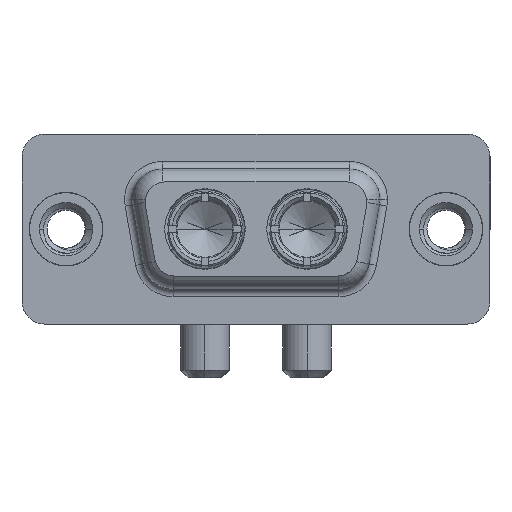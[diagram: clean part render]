
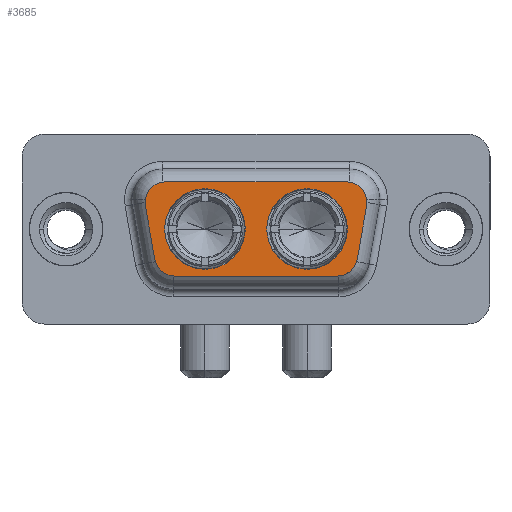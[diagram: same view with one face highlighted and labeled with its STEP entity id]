
A CAD part, top view. The second image highlights one B-rep face of the part: STEP entity #3685.
In plain terms, the highlighted planar face has unit normal (0, 0, 1).
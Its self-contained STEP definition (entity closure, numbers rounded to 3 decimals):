
#141 = CIRCLE ( 'NONE', #6974, 2.65 ) ;
#162 = VERTEX_POINT ( 'NONE', #2489 ) ;
#272 = EDGE_CURVE ( 'NONE', #11882, #10752, #141, .T. ) ;
#481 = AXIS2_PLACEMENT_3D ( 'NONE', #8998, #1704, #1577 ) ;
#513 = VERTEX_POINT ( 'NONE', #658 ) ;
#582 = EDGE_CURVE ( 'NONE', #7479, #8769, #7341, .T. ) ;
#658 = CARTESIAN_POINT ( 'NONE',  ( 17.833, -3.1, 6.2 ) ) ;
#794 = ORIENTED_EDGE ( 'NONE', *, *, #5328, .T. ) ;
#813 = EDGE_CURVE ( 'NONE', #10752, #11882, #9710, .T. ) ;
#940 = VERTEX_POINT ( 'NONE', #2238 ) ;
#1012 = CARTESIAN_POINT ( 'NONE',  ( 19.779, 1.516, 6.2 ) ) ;
#1133 = CARTESIAN_POINT ( 'NONE',  ( 6.55, 3.1, 6.2 ) ) ;
#1221 = EDGE_CURVE ( 'NONE', #513, #4350, #10902, .T. ) ;
#1240 = DIRECTION ( 'NONE',  ( 0., 0., 1. ) ) ;
#1475 = ORIENTED_EDGE ( 'NONE', *, *, #582, .T. ) ;
#1577 = DIRECTION ( 'NONE',  ( 1., 0., 0. ) ) ;
#1593 = LINE ( 'NONE', #2452, #9607 ) ;
#1704 = DIRECTION ( 'NONE',  ( 0., 0., 1. ) ) ;
#1776 = DIRECTION ( 'NONE',  ( -1., 0., 0. ) ) ;
#1839 = CARTESIAN_POINT ( 'NONE',  ( 19.162, -1.984, 6.2 ) ) ;
#2238 = CARTESIAN_POINT ( 'NONE',  ( 5.838, -1.984, 6.2 ) ) ;
#2259 = ORIENTED_EDGE ( 'NONE', *, *, #1221, .T. ) ;
#2313 = CARTESIAN_POINT ( 'NONE',  ( 18.51, 0., 6.2 ) ) ;
#2421 = AXIS2_PLACEMENT_3D ( 'NONE', #9107, #5480, #8126 ) ;
#2452 = CARTESIAN_POINT ( 'NONE',  ( 17.833, -3.1, 6.2 ) ) ;
#2489 = CARTESIAN_POINT ( 'NONE',  ( 5.221, 1.516, 6.2 ) ) ;
#2652 = CARTESIAN_POINT ( 'NONE',  ( 5.2, 1.75, 6.2 ) ) ;
#2676 = PLANE ( 'NONE',  #7298 ) ;
#2788 = CARTESIAN_POINT ( 'NONE',  ( 11.79, 0., 6.2 ) ) ;
#2874 = DIRECTION ( 'NONE',  ( 0., 0., 1. ) ) ;
#2906 = EDGE_CURVE ( 'NONE', #5602, #3617, #6152, .T. ) ;
#3051 = DIRECTION ( 'NONE',  ( 1., 0., 0. ) ) ;
#3231 = ORIENTED_EDGE ( 'NONE', *, *, #4166, .T. ) ;
#3270 = EDGE_LOOP ( 'NONE', ( #8296, #8407 ) ) ;
#3288 = CARTESIAN_POINT ( 'NONE',  ( 7.167, -3.1, 6.2 ) ) ;
#3304 = DIRECTION ( 'NONE',  ( 1., 0., 0. ) ) ;
#3306 = ORIENTED_EDGE ( 'NONE', *, *, #4454, .T. ) ;
#3411 = CARTESIAN_POINT ( 'NONE',  ( 7.167, -1.75, 6.2 ) ) ;
#3592 = AXIS2_PLACEMENT_3D ( 'NONE', #3713, #5357, #3051 ) ;
#3617 = VERTEX_POINT ( 'NONE', #2313 ) ;
#3652 = FACE_BOUND ( 'NONE', #3270, .T. ) ;
#3664 = EDGE_LOOP ( 'NONE', ( #5469, #6252 ) ) ;
#3685 = ADVANCED_FACE ( 'NONE', ( #3652, #12069, #4448 ), #2676, .F. ) ;
#3713 = CARTESIAN_POINT ( 'NONE',  ( 6.55, 1.75, 6.2 ) ) ;
#3870 = CARTESIAN_POINT ( 'NONE',  ( 17.833, -1.75, 6.2 ) ) ;
#3876 = CARTESIAN_POINT ( 'NONE',  ( 6.49, 0., 6.2 ) ) ;
#3910 = CIRCLE ( 'NONE', #6471, 1.35 ) ;
#4017 = CARTESIAN_POINT ( 'NONE',  ( 7.167, -1.75, 6.2 ) ) ;
#4047 = EDGE_CURVE ( 'NONE', #12054, #162, #3910, .T. ) ;
#4166 = EDGE_CURVE ( 'NONE', #10461, #513, #1593, .T. ) ;
#4350 = VERTEX_POINT ( 'NONE', #1839 ) ;
#4440 = VECTOR ( 'NONE', #9411, 1000. ) ;
#4448 = FACE_OUTER_BOUND ( 'NONE', #12048, .T. ) ;
#4454 = EDGE_CURVE ( 'NONE', #10345, #7479, #4959, .T. ) ;
#4733 = LINE ( 'NONE', #5910, #4936 ) ;
#4850 = CARTESIAN_POINT ( 'NONE',  ( 9.14, 0., 6.2 ) ) ;
#4936 = VECTOR ( 'NONE', #11373, 1000. ) ;
#4959 = CIRCLE ( 'NONE', #11833, 1.35 ) ;
#5169 = EDGE_CURVE ( 'NONE', #8769, #12054, #10083, .T. ) ;
#5328 = EDGE_CURVE ( 'NONE', #940, #10461, #8122, .T. ) ;
#5357 = DIRECTION ( 'NONE',  ( 0., 0., 1. ) ) ;
#5469 = ORIENTED_EDGE ( 'NONE', *, *, #813, .F. ) ;
#5480 = DIRECTION ( 'NONE',  ( 0., 0., 1. ) ) ;
#5495 = DIRECTION ( 'NONE',  ( -1., 0., 0. ) ) ;
#5602 = VERTEX_POINT ( 'NONE', #11368 ) ;
#5606 = DIRECTION ( 'NONE',  ( 0., 0., 1. ) ) ;
#5675 = LINE ( 'NONE', #1012, #4440 ) ;
#5910 = CARTESIAN_POINT ( 'NONE',  ( 5.838, -1.984, 6.2 ) ) ;
#6152 = CIRCLE ( 'NONE', #2421, 2.65 ) ;
#6164 = CIRCLE ( 'NONE', #481, 2.65 ) ;
#6240 = CARTESIAN_POINT ( 'NONE',  ( 6.55, 3.1, 6.2 ) ) ;
#6252 = ORIENTED_EDGE ( 'NONE', *, *, #272, .F. ) ;
#6471 = AXIS2_PLACEMENT_3D ( 'NONE', #7770, #10834, #10719 ) ;
#6670 = EDGE_CURVE ( 'NONE', #3617, #5602, #6164, .T. ) ;
#6714 = CARTESIAN_POINT ( 'NONE',  ( 9.14, 0., 6.2 ) ) ;
#6825 = DIRECTION ( 'NONE',  ( 1., 0., 0. ) ) ;
#6974 = AXIS2_PLACEMENT_3D ( 'NONE', #4850, #1240, #6825 ) ;
#7298 = AXIS2_PLACEMENT_3D ( 'NONE', #3411, #10911, #11156 ) ;
#7341 = LINE ( 'NONE', #6240, #8533 ) ;
#7479 = VERTEX_POINT ( 'NONE', #9886 ) ;
#7770 = CARTESIAN_POINT ( 'NONE',  ( 6.55, 1.75, 6.2 ) ) ;
#7778 = DIRECTION ( 'NONE',  ( 0., 0., 1. ) ) ;
#8122 = CIRCLE ( 'NONE', #10290, 1.35 ) ;
#8126 = DIRECTION ( 'NONE',  ( 1., 0., 0. ) ) ;
#8230 = ORIENTED_EDGE ( 'NONE', *, *, #5169, .T. ) ;
#8296 = ORIENTED_EDGE ( 'NONE', *, *, #6670, .F. ) ;
#8328 = DIRECTION ( 'NONE',  ( 1., 0., 0. ) ) ;
#8407 = ORIENTED_EDGE ( 'NONE', *, *, #2906, .F. ) ;
#8533 = VECTOR ( 'NONE', #5495, 1000. ) ;
#8769 = VERTEX_POINT ( 'NONE', #1133 ) ;
#8998 = CARTESIAN_POINT ( 'NONE',  ( 15.86, 0., 6.2 ) ) ;
#9107 = CARTESIAN_POINT ( 'NONE',  ( 15.86, 0., 6.2 ) ) ;
#9383 = ORIENTED_EDGE ( 'NONE', *, *, #4047, .T. ) ;
#9411 = DIRECTION ( 'NONE',  ( 0.174, 0.985, 0. ) ) ;
#9429 = CARTESIAN_POINT ( 'NONE',  ( 19.779, 1.516, 6.2 ) ) ;
#9451 = ORIENTED_EDGE ( 'NONE', *, *, #11742, .T. ) ;
#9488 = EDGE_CURVE ( 'NONE', #4350, #10345, #5675, .T. ) ;
#9607 = VECTOR ( 'NONE', #3304, 1000. ) ;
#9710 = CIRCLE ( 'NONE', #11280, 2.65 ) ;
#9722 = AXIS2_PLACEMENT_3D ( 'NONE', #3870, #5606, #11254 ) ;
#9886 = CARTESIAN_POINT ( 'NONE',  ( 18.45, 3.1, 6.2 ) ) ;
#10083 = CIRCLE ( 'NONE', #3592, 1.35 ) ;
#10290 = AXIS2_PLACEMENT_3D ( 'NONE', #4017, #7778, #11524 ) ;
#10345 = VERTEX_POINT ( 'NONE', #9429 ) ;
#10461 = VERTEX_POINT ( 'NONE', #3288 ) ;
#10477 = DIRECTION ( 'NONE',  ( 0., 0., 1. ) ) ;
#10719 = DIRECTION ( 'NONE',  ( 1., 0., 0. ) ) ;
#10752 = VERTEX_POINT ( 'NONE', #2788 ) ;
#10834 = DIRECTION ( 'NONE',  ( 0., 0., 1. ) ) ;
#10902 = CIRCLE ( 'NONE', #9722, 1.35 ) ;
#10911 = DIRECTION ( 'NONE',  ( 0., 0., -1. ) ) ;
#11116 = CARTESIAN_POINT ( 'NONE',  ( 18.45, 1.75, 6.2 ) ) ;
#11156 = DIRECTION ( 'NONE',  ( -1., 0., 0. ) ) ;
#11254 = DIRECTION ( 'NONE',  ( -1., 0., 0. ) ) ;
#11280 = AXIS2_PLACEMENT_3D ( 'NONE', #6714, #10477, #8328 ) ;
#11368 = CARTESIAN_POINT ( 'NONE',  ( 13.21, 0., 6.2 ) ) ;
#11373 = DIRECTION ( 'NONE',  ( 0.174, -0.985, 0. ) ) ;
#11524 = DIRECTION ( 'NONE',  ( -1., 0., 0. ) ) ;
#11686 = ORIENTED_EDGE ( 'NONE', *, *, #9488, .T. ) ;
#11742 = EDGE_CURVE ( 'NONE', #162, #940, #4733, .T. ) ;
#11833 = AXIS2_PLACEMENT_3D ( 'NONE', #11116, #2874, #1776 ) ;
#11882 = VERTEX_POINT ( 'NONE', #3876 ) ;
#12048 = EDGE_LOOP ( 'NONE', ( #794, #3231, #2259, #11686, #3306, #1475, #8230, #9383, #9451 ) ) ;
#12054 = VERTEX_POINT ( 'NONE', #2652 ) ;
#12069 = FACE_BOUND ( 'NONE', #3664, .T. ) ;
